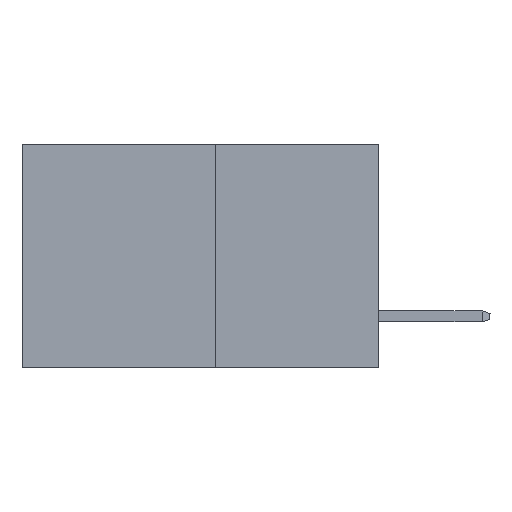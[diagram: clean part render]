
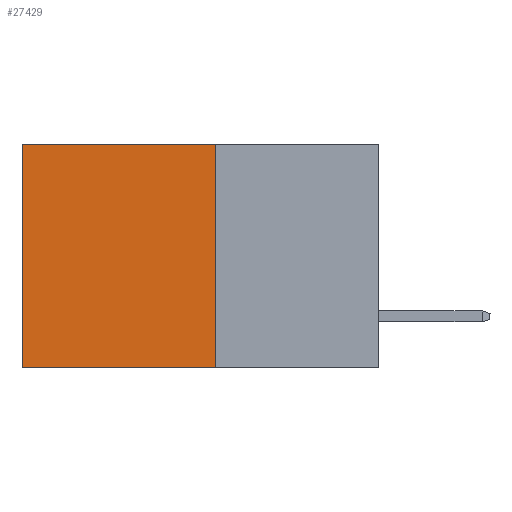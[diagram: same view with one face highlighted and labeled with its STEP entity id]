
A CAD part, left-side view. The second image highlights one B-rep face of the part: STEP entity #27429.
In plain terms, the highlighted planar face has unit normal (-1, 0, 0).
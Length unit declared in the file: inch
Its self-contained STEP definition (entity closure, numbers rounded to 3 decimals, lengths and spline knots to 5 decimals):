
#33 = CARTESIAN_POINT ( 'NONE',  ( 0.277, 0.27, 0. ) ) ;
#880 = CARTESIAN_POINT ( 'NONE',  ( 0.277, 0.27, -0.37 ) ) ;
#1456 = VECTOR ( 'NONE', #2819, 39.37008 ) ;
#2819 = DIRECTION ( 'NONE',  ( 0., 0., -1. ) ) ;
#4710 = ORIENTED_EDGE ( 'NONE', *, *, #17930, .T. ) ;
#5270 = EDGE_LOOP ( 'NONE', ( #13846, #23868, #23969, #4710 ) ) ;
#6228 = VERTEX_POINT ( 'NONE', #12457 ) ;
#6819 = PLANE ( 'NONE',  #29829 ) ;
#8973 = LINE ( 'NONE', #880, #28921 ) ;
#9100 = LINE ( 'NONE', #26033, #1456 ) ;
#9625 = EDGE_CURVE ( 'NONE', #6228, #29853, #9100, .T. ) ;
#11304 = EDGE_CURVE ( 'NONE', #27232, #21915, #8973, .T. ) ;
#12027 = CARTESIAN_POINT ( 'NONE',  ( 0.277, 0.27, -0.37 ) ) ;
#12457 = CARTESIAN_POINT ( 'NONE',  ( 0.277, 0.59, 0. ) ) ;
#12754 = LINE ( 'NONE', #33, #14395 ) ;
#13846 = ORIENTED_EDGE ( 'NONE', *, *, #9625, .T. ) ;
#13868 = CARTESIAN_POINT ( 'NONE',  ( 0.277, 0.27, 0. ) ) ;
#14395 = VECTOR ( 'NONE', #18127, 39.37008 ) ;
#14645 = DIRECTION ( 'NONE',  ( 0., 0., -1. ) ) ;
#16759 = CARTESIAN_POINT ( 'NONE',  ( 0.277, 0.27, -0.37 ) ) ;
#17930 = EDGE_CURVE ( 'NONE', #27232, #6228, #12754, .T. ) ;
#18127 = DIRECTION ( 'NONE',  ( 0., 1., 0. ) ) ;
#19359 = DIRECTION ( 'NONE',  ( 0., 1., 0. ) ) ;
#21605 = DIRECTION ( 'NONE',  ( 0., 0., -1. ) ) ;
#21915 = VERTEX_POINT ( 'NONE', #30228 ) ;
#22933 = EDGE_CURVE ( 'NONE', #21915, #29853, #33135, .T. ) ;
#23868 = ORIENTED_EDGE ( 'NONE', *, *, #22933, .F. ) ;
#23969 = ORIENTED_EDGE ( 'NONE', *, *, #11304, .F. ) ;
#25422 = VECTOR ( 'NONE', #19359, 39.37008 ) ;
#26021 = FACE_OUTER_BOUND ( 'NONE', #5270, .T. ) ;
#26033 = CARTESIAN_POINT ( 'NONE',  ( 0.277, 0.59, -0.37 ) ) ;
#27187 = CARTESIAN_POINT ( 'NONE',  ( 0.277, 0.59, -0.37 ) ) ;
#27232 = VERTEX_POINT ( 'NONE', #13868 ) ;
#27429 = ADVANCED_FACE ( 'NONE', ( #26021 ), #6819, .F. ) ;
#28921 = VECTOR ( 'NONE', #21605, 39.37008 ) ;
#29829 = AXIS2_PLACEMENT_3D ( 'NONE', #12027, #30203, #14645 ) ;
#29853 = VERTEX_POINT ( 'NONE', #27187 ) ;
#30203 = DIRECTION ( 'NONE',  ( 1., 0., 0. ) ) ;
#30228 = CARTESIAN_POINT ( 'NONE',  ( 0.277, 0.27, -0.37 ) ) ;
#33135 = LINE ( 'NONE', #16759, #25422 ) ;
